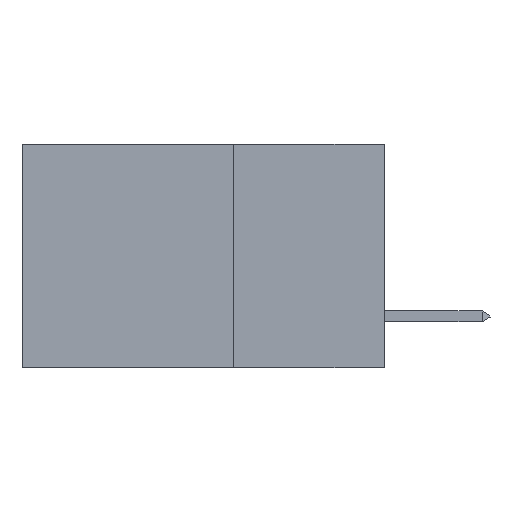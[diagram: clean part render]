
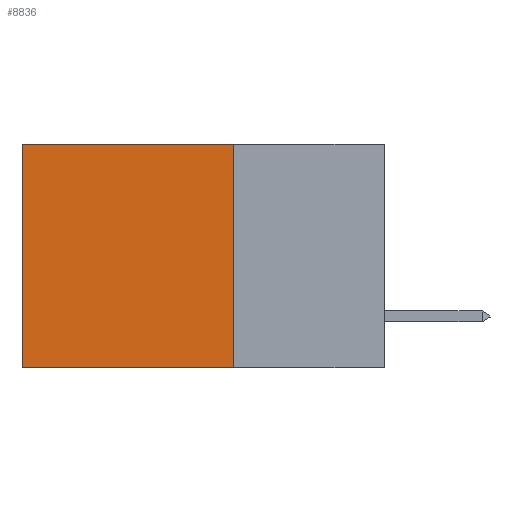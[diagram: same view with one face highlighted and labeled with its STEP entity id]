
A CAD part, left-side view. The second image highlights one B-rep face of the part: STEP entity #8836.
In plain terms, the highlighted planar face has unit normal (-1, 0, 0).
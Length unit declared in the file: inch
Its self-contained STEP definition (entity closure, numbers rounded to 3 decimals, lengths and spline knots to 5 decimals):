
#301 = VECTOR ( 'NONE', #7854, 39.37008 ) ;
#405 = ORIENTED_EDGE ( 'NONE', *, *, #8604, .F. ) ;
#716 = VECTOR ( 'NONE', #6416, 39.37008 ) ;
#796 = CARTESIAN_POINT ( 'NONE',  ( 0.2875, 0.6, 0. ) ) ;
#946 = DIRECTION ( 'NONE',  ( 1., 0., 0. ) ) ;
#1477 = CARTESIAN_POINT ( 'NONE',  ( 0.2875, 0.25, -0.37 ) ) ;
#1564 = DIRECTION ( 'NONE',  ( 0., 1., 0. ) ) ;
#1565 = LINE ( 'NONE', #8342, #301 ) ;
#2111 = LINE ( 'NONE', #9262, #716 ) ;
#2215 = EDGE_CURVE ( 'NONE', #4243, #5987, #1565, .T. ) ;
#2692 = CARTESIAN_POINT ( 'NONE',  ( 0.2875, 0.25, 0. ) ) ;
#3142 = EDGE_CURVE ( 'NONE', #5987, #5353, #6467, .T. ) ;
#3208 = PLANE ( 'NONE',  #7073 ) ;
#4243 = VERTEX_POINT ( 'NONE', #2692 ) ;
#4584 = CARTESIAN_POINT ( 'NONE',  ( 0.2875, 0.25, 0. ) ) ;
#4608 = DIRECTION ( 'NONE',  ( 0., 0., -1. ) ) ;
#5232 = DIRECTION ( 'NONE',  ( 0., 0., -1. ) ) ;
#5260 = VERTEX_POINT ( 'NONE', #1477 ) ;
#5353 = VERTEX_POINT ( 'NONE', #5504 ) ;
#5504 = CARTESIAN_POINT ( 'NONE',  ( 0.2875, 0.6, -0.37 ) ) ;
#5623 = FACE_OUTER_BOUND ( 'NONE', #6438, .T. ) ;
#5987 = VERTEX_POINT ( 'NONE', #7585 ) ;
#6416 = DIRECTION ( 'NONE',  ( 0., 0., -1. ) ) ;
#6438 = EDGE_LOOP ( 'NONE', ( #7992, #6701, #405, #7605 ) ) ;
#6467 = LINE ( 'NONE', #796, #8879 ) ;
#6623 = VECTOR ( 'NONE', #1564, 39.37008 ) ;
#6701 = ORIENTED_EDGE ( 'NONE', *, *, #7096, .F. ) ;
#6930 = LINE ( 'NONE', #7881, #6623 ) ;
#7073 = AXIS2_PLACEMENT_3D ( 'NONE', #4584, #946, #4608 ) ;
#7096 = EDGE_CURVE ( 'NONE', #5260, #5353, #6930, .T. ) ;
#7585 = CARTESIAN_POINT ( 'NONE',  ( 0.2875, 0.6, 0. ) ) ;
#7605 = ORIENTED_EDGE ( 'NONE', *, *, #2215, .T. ) ;
#7854 = DIRECTION ( 'NONE',  ( 0., 1., 0. ) ) ;
#7881 = CARTESIAN_POINT ( 'NONE',  ( 0.2875, 0.25, -0.37 ) ) ;
#7992 = ORIENTED_EDGE ( 'NONE', *, *, #3142, .T. ) ;
#8342 = CARTESIAN_POINT ( 'NONE',  ( 0.2875, 0.25, 0. ) ) ;
#8604 = EDGE_CURVE ( 'NONE', #4243, #5260, #2111, .T. ) ;
#8836 = ADVANCED_FACE ( 'NONE', ( #5623 ), #3208, .F. ) ;
#8879 = VECTOR ( 'NONE', #5232, 39.37008 ) ;
#9262 = CARTESIAN_POINT ( 'NONE',  ( 0.2875, 0.25, 0. ) ) ;
